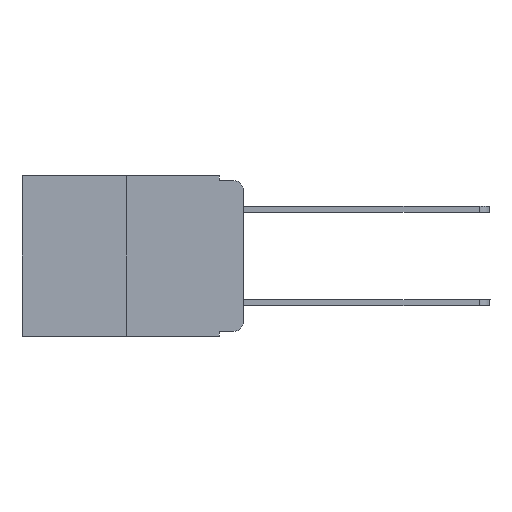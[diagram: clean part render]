
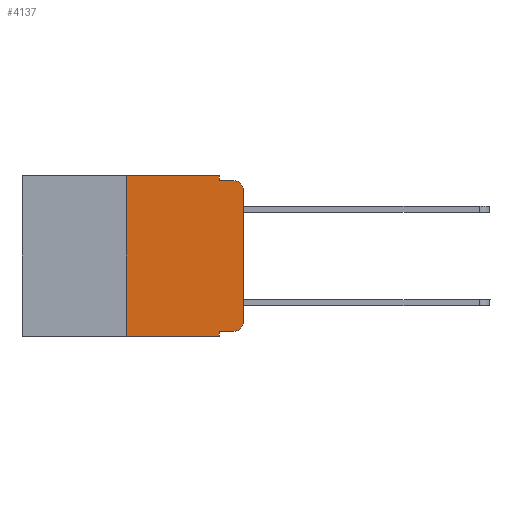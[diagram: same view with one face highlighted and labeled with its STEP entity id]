
A CAD part, left-side view. The second image highlights one B-rep face of the part: STEP entity #4137.
In plain terms, the highlighted planar face has unit normal (-1, 0, 0).
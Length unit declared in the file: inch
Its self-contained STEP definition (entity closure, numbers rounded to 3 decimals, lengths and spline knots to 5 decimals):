
#111 = DIRECTION ( 'NONE',  ( 0., 0., -1. ) ) ;
#149 = VECTOR ( 'NONE', #4379, 39.37008 ) ;
#480 = LINE ( 'NONE', #3840, #13438 ) ;
#611 = CARTESIAN_POINT ( 'NONE',  ( 0., 0.473, 0. ) ) ;
#780 = VERTEX_POINT ( 'NONE', #7039 ) ;
#1118 = CARTESIAN_POINT ( 'NONE',  ( 0., 0.051, 0. ) ) ;
#1126 = ORIENTED_EDGE ( 'NONE', *, *, #1214, .F. ) ;
#1214 = EDGE_CURVE ( 'NONE', #15905, #8777, #16389, .T. ) ;
#1787 = CARTESIAN_POINT ( 'NONE',  ( 0., 0.051, -0.343 ) ) ;
#1811 = CARTESIAN_POINT ( 'NONE',  ( 0., 0.25, 0. ) ) ;
#1857 = CARTESIAN_POINT ( 'NONE',  ( 0., 0.473, 0. ) ) ;
#1928 = DIRECTION ( 'NONE',  ( 0., -1., 0. ) ) ;
#1954 = EDGE_CURVE ( 'NONE', #11796, #3682, #10530, .T. ) ;
#2526 = CARTESIAN_POINT ( 'NONE',  ( 0., 0.02, -0.313 ) ) ;
#2564 = DIRECTION ( 'NONE',  ( 0., 0., -1. ) ) ;
#2978 = DIRECTION ( 'NONE',  ( -1., 0., 0. ) ) ;
#3029 = AXIS2_PLACEMENT_3D ( 'NONE', #2526, #11257, #9775 ) ;
#3134 = DIRECTION ( 'NONE',  ( 0., -1., 0. ) ) ;
#3211 = LINE ( 'NONE', #6253, #17621 ) ;
#3337 = AXIS2_PLACEMENT_3D ( 'NONE', #7586, #2978, #111 ) ;
#3520 = CARTESIAN_POINT ( 'NONE',  ( 0., 0.02, -0.333 ) ) ;
#3582 = ORIENTED_EDGE ( 'NONE', *, *, #14498, .F. ) ;
#3682 = VERTEX_POINT ( 'NONE', #4472 ) ;
#3795 = LINE ( 'NONE', #8483, #12892 ) ;
#3840 = CARTESIAN_POINT ( 'NONE',  ( 0., 0., 0. ) ) ;
#4040 = CARTESIAN_POINT ( 'NONE',  ( 0., 0.051, 0. ) ) ;
#4137 = ADVANCED_FACE ( 'NONE', ( #5444 ), #9732, .F. ) ;
#4379 = DIRECTION ( 'NONE',  ( 0., 0., 1. ) ) ;
#4472 = CARTESIAN_POINT ( 'NONE',  ( 0., 0., -0.313 ) ) ;
#4481 = CARTESIAN_POINT ( 'NONE',  ( 0., 0.02, -0.01 ) ) ;
#4552 = CARTESIAN_POINT ( 'NONE',  ( 0., 0.25, -0.343 ) ) ;
#5444 = FACE_OUTER_BOUND ( 'NONE', #11918, .T. ) ;
#5847 = CIRCLE ( 'NONE', #3337, 0.02 ) ;
#5862 = CARTESIAN_POINT ( 'NONE',  ( 0., 0.051, -0.01 ) ) ;
#6129 = EDGE_CURVE ( 'NONE', #15329, #11897, #13138, .T. ) ;
#6253 = CARTESIAN_POINT ( 'NONE',  ( 0., 0.473, -0.343 ) ) ;
#6988 = VECTOR ( 'NONE', #10868, 39.37008 ) ;
#7039 = CARTESIAN_POINT ( 'NONE',  ( 0., 0., -0.03 ) ) ;
#7396 = ORIENTED_EDGE ( 'NONE', *, *, #16110, .T. ) ;
#7544 = EDGE_CURVE ( 'NONE', #780, #8460, #5847, .T. ) ;
#7586 = CARTESIAN_POINT ( 'NONE',  ( 0., 0.02, -0.03 ) ) ;
#7790 = LINE ( 'NONE', #1811, #149 ) ;
#8049 = DIRECTION ( 'NONE',  ( 0., 0., 1. ) ) ;
#8338 = ORIENTED_EDGE ( 'NONE', *, *, #7544, .T. ) ;
#8460 = VERTEX_POINT ( 'NONE', #4481 ) ;
#8483 = CARTESIAN_POINT ( 'NONE',  ( 0., 0.051, -0.01 ) ) ;
#8777 = VERTEX_POINT ( 'NONE', #1787 ) ;
#9135 = VECTOR ( 'NONE', #16107, 39.37008 ) ;
#9290 = LINE ( 'NONE', #1857, #6988 ) ;
#9319 = AXIS2_PLACEMENT_3D ( 'NONE', #611, #14238, #12570 ) ;
#9732 = PLANE ( 'NONE',  #9319 ) ;
#9775 = DIRECTION ( 'NONE',  ( 0., 0., -1. ) ) ;
#9846 = DIRECTION ( 'NONE',  ( 0., -1., 0. ) ) ;
#9951 = ORIENTED_EDGE ( 'NONE', *, *, #15630, .F. ) ;
#10198 = CARTESIAN_POINT ( 'NONE',  ( 0., 0.051, 0. ) ) ;
#10310 = ORIENTED_EDGE ( 'NONE', *, *, #12682, .T. ) ;
#10384 = EDGE_CURVE ( 'NONE', #15905, #11796, #10563, .T. ) ;
#10530 = CIRCLE ( 'NONE', #3029, 0.02 ) ;
#10563 = LINE ( 'NONE', #16534, #11205 ) ;
#10756 = VERTEX_POINT ( 'NONE', #4552 ) ;
#10868 = DIRECTION ( 'NONE',  ( 0., -1., 0. ) ) ;
#11205 = VECTOR ( 'NONE', #3134, 39.37008 ) ;
#11257 = DIRECTION ( 'NONE',  ( -1., 0., 0. ) ) ;
#11414 = CARTESIAN_POINT ( 'NONE',  ( 0., 0.25, 0. ) ) ;
#11796 = VERTEX_POINT ( 'NONE', #3520 ) ;
#11897 = VERTEX_POINT ( 'NONE', #5862 ) ;
#11918 = EDGE_LOOP ( 'NONE', ( #10310, #8338, #3582, #12125, #9951, #14640, #7396, #1126, #18089, #18156 ) ) ;
#12125 = ORIENTED_EDGE ( 'NONE', *, *, #6129, .F. ) ;
#12570 = DIRECTION ( 'NONE',  ( 0., 0., -1. ) ) ;
#12682 = EDGE_CURVE ( 'NONE', #3682, #780, #480, .T. ) ;
#12892 = VECTOR ( 'NONE', #9846, 39.37008 ) ;
#12992 = VECTOR ( 'NONE', #2564, 39.37008 ) ;
#13138 = LINE ( 'NONE', #10198, #12992 ) ;
#13198 = VERTEX_POINT ( 'NONE', #11414 ) ;
#13438 = VECTOR ( 'NONE', #8049, 39.37008 ) ;
#14238 = DIRECTION ( 'NONE',  ( 1., 0., 0. ) ) ;
#14498 = EDGE_CURVE ( 'NONE', #11897, #8460, #3795, .T. ) ;
#14640 = ORIENTED_EDGE ( 'NONE', *, *, #18103, .F. ) ;
#15329 = VERTEX_POINT ( 'NONE', #4040 ) ;
#15630 = EDGE_CURVE ( 'NONE', #13198, #15329, #9290, .T. ) ;
#15905 = VERTEX_POINT ( 'NONE', #18985 ) ;
#16107 = DIRECTION ( 'NONE',  ( 0., 0., -1. ) ) ;
#16110 = EDGE_CURVE ( 'NONE', #10756, #8777, #3211, .T. ) ;
#16389 = LINE ( 'NONE', #1118, #9135 ) ;
#16534 = CARTESIAN_POINT ( 'NONE',  ( 0., 0.051, -0.333 ) ) ;
#17621 = VECTOR ( 'NONE', #1928, 39.37008 ) ;
#18089 = ORIENTED_EDGE ( 'NONE', *, *, #10384, .T. ) ;
#18103 = EDGE_CURVE ( 'NONE', #10756, #13198, #7790, .T. ) ;
#18156 = ORIENTED_EDGE ( 'NONE', *, *, #1954, .T. ) ;
#18985 = CARTESIAN_POINT ( 'NONE',  ( 0., 0.051, -0.333 ) ) ;
